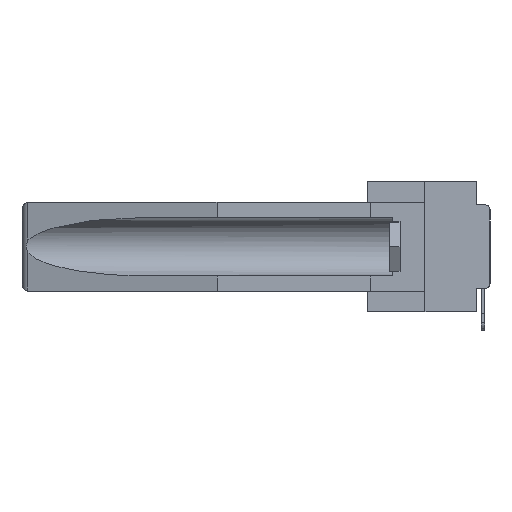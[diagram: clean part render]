
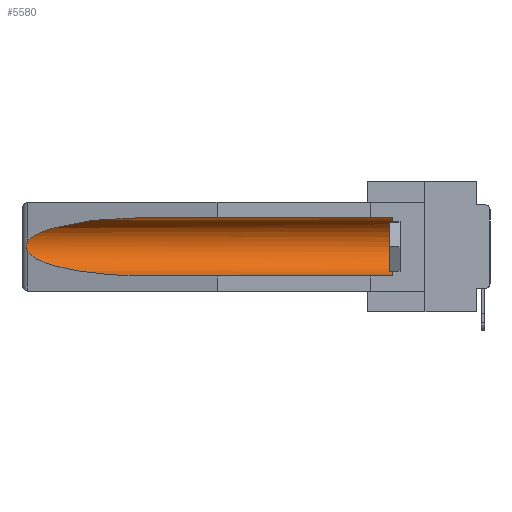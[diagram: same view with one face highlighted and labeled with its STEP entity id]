
A CAD part, left-side view. The second image highlights one B-rep face of the part: STEP entity #5580.
In plain terms, the highlighted cylindrical face has radius 2.857 mm (diameter 5.715 mm), a partial arc.
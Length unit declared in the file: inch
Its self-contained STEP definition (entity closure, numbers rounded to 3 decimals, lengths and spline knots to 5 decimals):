
#460 = CARTESIAN_POINT ( 'NONE',  ( 0.26655, 1.53094, -0.18657 ) ) ;
#602 = EDGE_CURVE ( 'NONE', #13612, #4777, #14549, .T. ) ;
#986 = DIRECTION ( 'NONE',  ( 0., 0., 1. ) ) ;
#2650 = ORIENTED_EDGE ( 'NONE', *, *, #23652, .T. ) ;
#2893 = CARTESIAN_POINT ( 'NONE',  ( 0.2673, 1.5327, -0.16383 ) ) ;
#3579 = DIRECTION ( 'NONE',  ( 0., 1., 0. ) ) ;
#4502 = EDGE_LOOP ( 'NONE', ( #11855, #16616, #11012, #7337, #2650, #7720 ) ) ;
#4777 = VERTEX_POINT ( 'NONE', #32858 ) ;
#4815 = CARTESIAN_POINT ( 'NONE',  ( 0.155, 0.126, -0.284 ) ) ;
#5049 = DIRECTION ( 'NONE',  ( 0., 1., 0. ) ) ;
#5389 = CARTESIAN_POINT ( 'NONE',  ( 0.155, -0.30754, -0.059 ) ) ;
#5520 = CARTESIAN_POINT ( 'NONE',  ( 0.26597, 1.52961, -0.15275 ) ) ;
#5580 = ADVANCED_FACE ( 'NONE', ( #9614 ), #35225, .F. ) ;
#5726 = CARTESIAN_POINT ( 'NONE',  ( 0.2673, 1.53269, -0.17917 ) ) ;
#5801 = EDGE_CURVE ( 'NONE', #18849, #22900, #36875, .T. ) ;
#6064 = CARTESIAN_POINT ( 'NONE',  ( 0.26537, 1.52718, -0.19328 ) ) ;
#6411 = CARTESIAN_POINT ( 'NONE',  ( 0.155, -0.30754, -0.1715 ) ) ;
#7264 = AXIS2_PLACEMENT_3D ( 'NONE', #6411, #3579, #29548 ) ;
#7310 =( BOUNDED_CURVE ( )  B_SPLINE_CURVE ( 3, ( #6064, #14930, #29413, #23614 ),
 .UNSPECIFIED., .F., .T. ) 
 B_SPLINE_CURVE_WITH_KNOTS ( ( 4, 4 ),
 ( 0.1948, 1.5708 ),
 .UNSPECIFIED. ) 
 CURVE ( )  GEOMETRIC_REPRESENTATION_ITEM ( )  RATIONAL_B_SPLINE_CURVE ( ( 1., 0.848, 0.848, 1. ) ) 
 REPRESENTATION_ITEM ( '' )  );
#7337 = ORIENTED_EDGE ( 'NONE', *, *, #5801, .F. ) ;
#7409 = AXIS2_PLACEMENT_3D ( 'NONE', #26598, #20970, #986 ) ;
#7720 = ORIENTED_EDGE ( 'NONE', *, *, #34762, .T. ) ;
#9614 = FACE_OUTER_BOUND ( 'NONE', #4502, .T. ) ;
#10328 = VECTOR ( 'NONE', #5049, 39.37008 ) ;
#10608 = EDGE_CURVE ( 'NONE', #17693, #13612, #24950, .T. ) ;
#11012 = ORIENTED_EDGE ( 'NONE', *, *, #24958, .T. ) ;
#11133 = CARTESIAN_POINT ( 'NONE',  ( 0.155, 1.07973, -0.059 ) ) ;
#11489 = CARTESIAN_POINT ( 'NONE',  ( 0.25451, 1.48313, -0.09465 ) ) ;
#11565 = CARTESIAN_POINT ( 'NONE',  ( 0.26597, 1.5296, -0.19026 ) ) ;
#11855 = ORIENTED_EDGE ( 'NONE', *, *, #10608, .T. ) ;
#13612 = VERTEX_POINT ( 'NONE', #31277 ) ;
#14257 = LINE ( 'NONE', #5389, #24499 ) ;
#14549 = B_SPLINE_CURVE_WITH_KNOTS ( 'NONE', 3,
 ( #34335, #5520, #25534, #2893, #14776, #36995, #5726, #460, #11565, #22718 ),
 .UNSPECIFIED., .F., .F.,
 ( 4, 2, 2, 2, 4 ),
 ( 0., 0.00029, 0.00058, 0.00087, 0.00117 ),
 .UNSPECIFIED. ) ;
#14776 = CARTESIAN_POINT ( 'NONE',  ( 0.2675, 1.53308, -0.16763 ) ) ;
#14930 = CARTESIAN_POINT ( 'NONE',  ( 0.25451, 1.48313, -0.24835 ) ) ;
#16616 = ORIENTED_EDGE ( 'NONE', *, *, #602, .T. ) ;
#17152 = CARTESIAN_POINT ( 'NONE',  ( 0.26537, 1.52718, -0.14972 ) ) ;
#17693 = VERTEX_POINT ( 'NONE', #33815 ) ;
#18849 = VERTEX_POINT ( 'NONE', #4815 ) ;
#20970 = DIRECTION ( 'NONE',  ( 0., -1., 0. ) ) ;
#22142 = CARTESIAN_POINT ( 'NONE',  ( 0.155, 1.07973, -0.284 ) ) ;
#22610 = CARTESIAN_POINT ( 'NONE',  ( 0.155, -0.30754, -0.284 ) ) ;
#22718 = CARTESIAN_POINT ( 'NONE',  ( 0.26537, 1.52718, -0.19328 ) ) ;
#22900 = VERTEX_POINT ( 'NONE', #22142 ) ;
#23582 = CARTESIAN_POINT ( 'NONE',  ( 0.155, 0.126, -0.059 ) ) ;
#23614 = CARTESIAN_POINT ( 'NONE',  ( 0.155, 1.07973, -0.284 ) ) ;
#23652 = EDGE_CURVE ( 'NONE', #18849, #31068, #35072, .T. ) ;
#24499 = VECTOR ( 'NONE', #31196, 39.37008 ) ;
#24950 =( BOUNDED_CURVE ( )  B_SPLINE_CURVE ( 3, ( #11133, #34830, #11489, #17152 ),
 .UNSPECIFIED., .F., .T. ) 
 B_SPLINE_CURVE_WITH_KNOTS ( ( 4, 4 ),
 ( 4.71239, 6.08839 ),
 .UNSPECIFIED. ) 
 CURVE ( )  GEOMETRIC_REPRESENTATION_ITEM ( )  RATIONAL_B_SPLINE_CURVE ( ( 1., 0.848, 0.848, 1. ) ) 
 REPRESENTATION_ITEM ( '' )  );
#24958 = EDGE_CURVE ( 'NONE', #4777, #22900, #7310, .T. ) ;
#25534 = CARTESIAN_POINT ( 'NONE',  ( 0.26654, 1.53092, -0.15636 ) ) ;
#26598 = CARTESIAN_POINT ( 'NONE',  ( 0.155, 0.126, -0.1715 ) ) ;
#29413 = CARTESIAN_POINT ( 'NONE',  ( 0.21114, 1.30732, -0.284 ) ) ;
#29548 = DIRECTION ( 'NONE',  ( 0., 0., 1. ) ) ;
#31068 = VERTEX_POINT ( 'NONE', #23582 ) ;
#31196 = DIRECTION ( 'NONE',  ( 0., 1., 0. ) ) ;
#31277 = CARTESIAN_POINT ( 'NONE',  ( 0.26537, 1.52718, -0.14972 ) ) ;
#32858 = CARTESIAN_POINT ( 'NONE',  ( 0.26537, 1.52718, -0.19328 ) ) ;
#33815 = CARTESIAN_POINT ( 'NONE',  ( 0.155, 1.07973, -0.059 ) ) ;
#34335 = CARTESIAN_POINT ( 'NONE',  ( 0.26537, 1.52718, -0.14972 ) ) ;
#34762 = EDGE_CURVE ( 'NONE', #31068, #17693, #14257, .T. ) ;
#34830 = CARTESIAN_POINT ( 'NONE',  ( 0.21114, 1.30732, -0.059 ) ) ;
#35072 = CIRCLE ( 'NONE', #7409, 0.1125 ) ;
#35225 = CYLINDRICAL_SURFACE ( 'NONE', #7264, 0.1125 ) ;
#36875 = LINE ( 'NONE', #22610, #10328 ) ;
#36995 = CARTESIAN_POINT ( 'NONE',  ( 0.2675, 1.53308, -0.17534 ) ) ;
